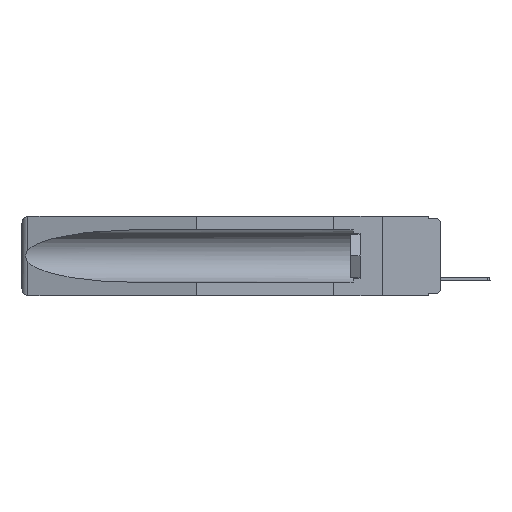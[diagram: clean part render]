
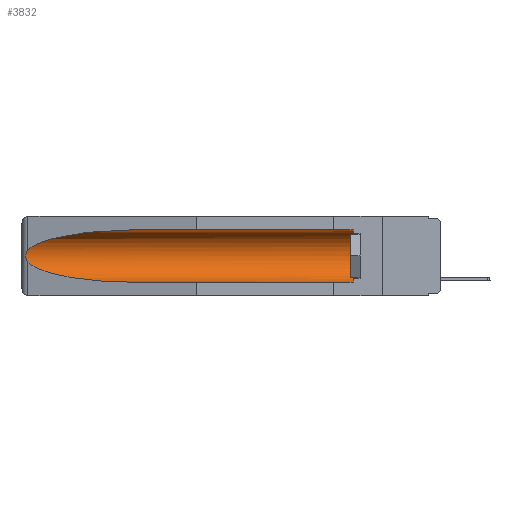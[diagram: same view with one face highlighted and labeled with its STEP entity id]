
A CAD part, left-side view. The second image highlights one B-rep face of the part: STEP entity #3832.
In plain terms, the highlighted cylindrical face has radius 2.857 mm (diameter 5.715 mm), a partial arc.
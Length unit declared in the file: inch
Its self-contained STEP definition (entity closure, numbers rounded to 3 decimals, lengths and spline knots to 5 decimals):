
#21 = CARTESIAN_POINT ( 'NONE',  ( 0.26597, 1.5296, -0.19026 ) ) ;
#198 = ORIENTED_EDGE ( 'NONE', *, *, #26040, .T. ) ;
#269 = ORIENTED_EDGE ( 'NONE', *, *, #6578, .F. ) ;
#720 = CARTESIAN_POINT ( 'NONE',  ( 0.26537, 1.52718, -0.14972 ) ) ;
#1053 = CARTESIAN_POINT ( 'NONE',  ( 0.155, 1.07973, -0.284 ) ) ;
#1692 = VECTOR ( 'NONE', #9701, 39.37008 ) ;
#3620 = CARTESIAN_POINT ( 'NONE',  ( 0.155, -0.30754, -0.1715 ) ) ;
#3832 = ADVANCED_FACE ( 'NONE', ( #21376 ), #8756, .F. ) ;
#3917 = AXIS2_PLACEMENT_3D ( 'NONE', #14102, #7748, #15883 ) ;
#4186 = CARTESIAN_POINT ( 'NONE',  ( 0.2673, 1.53269, -0.17917 ) ) ;
#4972 = CARTESIAN_POINT ( 'NONE',  ( 0.26537, 1.52718, -0.19328 ) ) ;
#5229 = ORIENTED_EDGE ( 'NONE', *, *, #26927, .T. ) ;
#5822 = CARTESIAN_POINT ( 'NONE',  ( 0.155, 0.126, -0.059 ) ) ;
#5982 = LINE ( 'NONE', #7277, #1692 ) ;
#6578 = EDGE_CURVE ( 'NONE', #11183, #9728, #23216, .T. ) ;
#7104 = CARTESIAN_POINT ( 'NONE',  ( 0.26537, 1.52718, -0.14972 ) ) ;
#7277 = CARTESIAN_POINT ( 'NONE',  ( 0.155, -0.30754, -0.059 ) ) ;
#7369 = CARTESIAN_POINT ( 'NONE',  ( 0.25451, 1.48313, -0.09465 ) ) ;
#7748 = DIRECTION ( 'NONE',  ( 0., -1., 0. ) ) ;
#8371 = CARTESIAN_POINT ( 'NONE',  ( 0.2675, 1.53308, -0.16763 ) ) ;
#8756 = CYLINDRICAL_SURFACE ( 'NONE', #14832, 0.1125 ) ;
#8764 = EDGE_LOOP ( 'NONE', ( #21182, #198, #5229, #269, #23672, #26121 ) ) ;
#9615 = EDGE_CURVE ( 'NONE', #18542, #20067, #15989, .T. ) ;
#9701 = DIRECTION ( 'NONE',  ( 0., 1., 0. ) ) ;
#9728 = VERTEX_POINT ( 'NONE', #1053 ) ;
#10512 = CARTESIAN_POINT ( 'NONE',  ( 0.26597, 1.52961, -0.15275 ) ) ;
#10691 = CARTESIAN_POINT ( 'NONE',  ( 0.2675, 1.53308, -0.17534 ) ) ;
#11019 = CARTESIAN_POINT ( 'NONE',  ( 0.21114, 1.30732, -0.284 ) ) ;
#11183 = VERTEX_POINT ( 'NONE', #20085 ) ;
#11790 = DIRECTION ( 'NONE',  ( 0., 1., 0. ) ) ;
#12630 = VECTOR ( 'NONE', #22999, 39.37008 ) ;
#13087 = B_SPLINE_CURVE_WITH_KNOTS ( 'NONE', 3,
 ( #27408, #10512, #16926, #15061, #8371, #10691, #4186, #25477, #21, #25558 ),
 .UNSPECIFIED., .F., .F.,
 ( 4, 2, 2, 2, 4 ),
 ( 0., 0.00029, 0.00058, 0.00087, 0.00117 ),
 .UNSPECIFIED. ) ;
#14102 = CARTESIAN_POINT ( 'NONE',  ( 0.155, 0.126, -0.1715 ) ) ;
#14832 = AXIS2_PLACEMENT_3D ( 'NONE', #3620, #11790, #26745 ) ;
#14944 = CARTESIAN_POINT ( 'NONE',  ( 0.26537, 1.52718, -0.19328 ) ) ;
#15061 = CARTESIAN_POINT ( 'NONE',  ( 0.2673, 1.5327, -0.16383 ) ) ;
#15304 = CARTESIAN_POINT ( 'NONE',  ( 0.155, 1.07973, -0.284 ) ) ;
#15883 = DIRECTION ( 'NONE',  ( 0., 0., 1. ) ) ;
#15989 =( BOUNDED_CURVE ( )  B_SPLINE_CURVE ( 3, ( #22149, #24340, #7369, #7104 ),
 .UNSPECIFIED., .F., .F. ) 
 B_SPLINE_CURVE_WITH_KNOTS ( ( 4, 4 ),
 ( 4.71239, 6.08839 ),
 .UNSPECIFIED. ) 
 CURVE ( )  GEOMETRIC_REPRESENTATION_ITEM ( )  RATIONAL_B_SPLINE_CURVE ( ( 1., 0.848, 0.848, 1. ) ) 
 REPRESENTATION_ITEM ( '' )  );
#16771 = CIRCLE ( 'NONE', #3917, 0.1125 ) ;
#16926 = CARTESIAN_POINT ( 'NONE',  ( 0.26654, 1.53092, -0.15636 ) ) ;
#17793 = CARTESIAN_POINT ( 'NONE',  ( 0.25451, 1.48313, -0.24835 ) ) ;
#18326 = CARTESIAN_POINT ( 'NONE',  ( 0.155, 1.07973, -0.059 ) ) ;
#18542 = VERTEX_POINT ( 'NONE', #18326 ) ;
#20067 = VERTEX_POINT ( 'NONE', #720 ) ;
#20085 = CARTESIAN_POINT ( 'NONE',  ( 0.155, 0.126, -0.284 ) ) ;
#21182 = ORIENTED_EDGE ( 'NONE', *, *, #9615, .T. ) ;
#21376 = FACE_OUTER_BOUND ( 'NONE', #8764, .T. ) ;
#21839 = EDGE_CURVE ( 'NONE', #11183, #26408, #16771, .T. ) ;
#22149 = CARTESIAN_POINT ( 'NONE',  ( 0.155, 1.07973, -0.059 ) ) ;
#22999 = DIRECTION ( 'NONE',  ( 0., 1., 0. ) ) ;
#23216 = LINE ( 'NONE', #25103, #12630 ) ;
#23672 = ORIENTED_EDGE ( 'NONE', *, *, #21839, .T. ) ;
#24340 = CARTESIAN_POINT ( 'NONE',  ( 0.21114, 1.30732, -0.059 ) ) ;
#24942 =( BOUNDED_CURVE ( )  B_SPLINE_CURVE ( 3, ( #4972, #17793, #11019, #15304 ),
 .UNSPECIFIED., .F., .F. ) 
 B_SPLINE_CURVE_WITH_KNOTS ( ( 4, 4 ),
 ( 0.1948, 1.5708 ),
 .UNSPECIFIED. ) 
 CURVE ( )  GEOMETRIC_REPRESENTATION_ITEM ( )  RATIONAL_B_SPLINE_CURVE ( ( 1., 0.848, 0.848, 1. ) ) 
 REPRESENTATION_ITEM ( '' )  );
#25103 = CARTESIAN_POINT ( 'NONE',  ( 0.155, -0.30754, -0.284 ) ) ;
#25477 = CARTESIAN_POINT ( 'NONE',  ( 0.26655, 1.53094, -0.18657 ) ) ;
#25558 = CARTESIAN_POINT ( 'NONE',  ( 0.26537, 1.52718, -0.19328 ) ) ;
#26040 = EDGE_CURVE ( 'NONE', #20067, #26763, #13087, .T. ) ;
#26121 = ORIENTED_EDGE ( 'NONE', *, *, #27100, .T. ) ;
#26408 = VERTEX_POINT ( 'NONE', #5822 ) ;
#26745 = DIRECTION ( 'NONE',  ( 0., 0., 1. ) ) ;
#26763 = VERTEX_POINT ( 'NONE', #14944 ) ;
#26927 = EDGE_CURVE ( 'NONE', #26763, #9728, #24942, .T. ) ;
#27100 = EDGE_CURVE ( 'NONE', #26408, #18542, #5982, .T. ) ;
#27408 = CARTESIAN_POINT ( 'NONE',  ( 0.26537, 1.52718, -0.14972 ) ) ;
